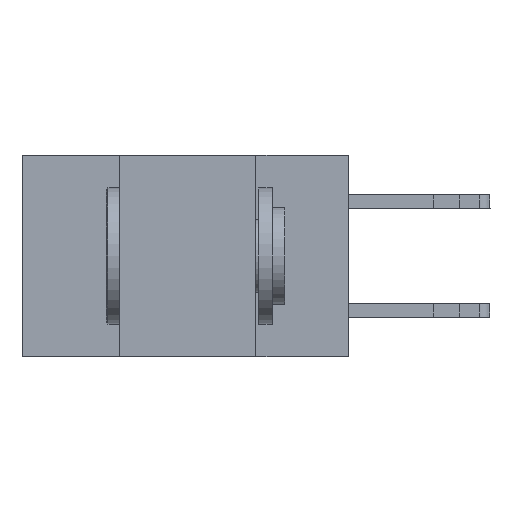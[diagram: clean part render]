
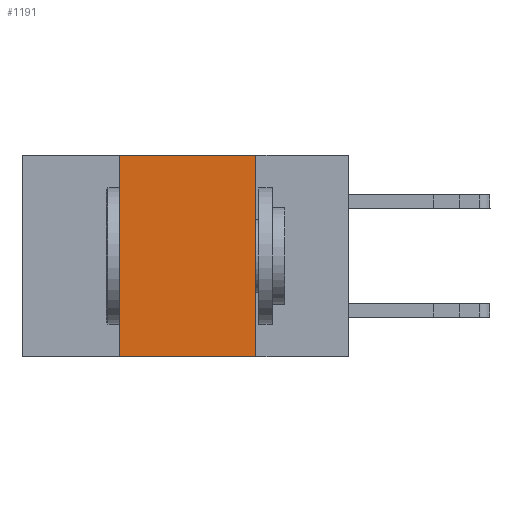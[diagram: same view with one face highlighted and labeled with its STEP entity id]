
A CAD part, left-side view. The second image highlights one B-rep face of the part: STEP entity #1191.
In plain terms, the highlighted planar face has unit normal (-1, 0, 0).
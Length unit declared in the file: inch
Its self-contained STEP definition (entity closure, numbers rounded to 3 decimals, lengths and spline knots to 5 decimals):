
#164 = ORIENTED_EDGE ( 'NONE', *, *, #8032, .T. ) ;
#178 = ORIENTED_EDGE ( 'NONE', *, *, #5772, .F. ) ;
#210 = CARTESIAN_POINT ( 'NONE',  ( 0., 0.6, 0. ) ) ;
#776 = CARTESIAN_POINT ( 'NONE',  ( 0., 0.6, 0. ) ) ;
#1191 = ADVANCED_FACE ( 'NONE', ( #9233 ), #8051, .F. ) ;
#1255 = VECTOR ( 'NONE', #7173, 39.37008 ) ;
#1764 = LINE ( 'NONE', #10640, #3026 ) ;
#2002 = VECTOR ( 'NONE', #3952, 39.37008 ) ;
#2213 = DIRECTION ( 'NONE',  ( 0., 0., -1. ) ) ;
#2550 = LINE ( 'NONE', #6993, #9428 ) ;
#2811 = CARTESIAN_POINT ( 'NONE',  ( 0., 0.17, -0.37 ) ) ;
#2927 = EDGE_LOOP ( 'NONE', ( #6967, #178, #12974, #164 ) ) ;
#3026 = VECTOR ( 'NONE', #9819, 39.37008 ) ;
#3538 = DIRECTION ( 'NONE',  ( 1., 0., 0. ) ) ;
#3952 = DIRECTION ( 'NONE',  ( 0., -1., 0. ) ) ;
#4082 = AXIS2_PLACEMENT_3D ( 'NONE', #210, #3538, #2213 ) ;
#4520 = EDGE_CURVE ( 'NONE', #13511, #6737, #2550, .T. ) ;
#5772 = EDGE_CURVE ( 'NONE', #6536, #13511, #12866, .T. ) ;
#5846 = CARTESIAN_POINT ( 'NONE',  ( 0., 0.42, 0. ) ) ;
#6536 = VERTEX_POINT ( 'NONE', #5846 ) ;
#6737 = VERTEX_POINT ( 'NONE', #2811 ) ;
#6967 = ORIENTED_EDGE ( 'NONE', *, *, #4520, .F. ) ;
#6993 = CARTESIAN_POINT ( 'NONE',  ( 0., 0.17, 0. ) ) ;
#7173 = DIRECTION ( 'NONE',  ( 0., -1., 0. ) ) ;
#8032 = EDGE_CURVE ( 'NONE', #10723, #6737, #9033, .T. ) ;
#8051 = PLANE ( 'NONE',  #4082 ) ;
#9033 = LINE ( 'NONE', #13518, #1255 ) ;
#9233 = FACE_OUTER_BOUND ( 'NONE', #2927, .T. ) ;
#9428 = VECTOR ( 'NONE', #12586, 39.37008 ) ;
#9819 = DIRECTION ( 'NONE',  ( 0., 0., 1. ) ) ;
#10640 = CARTESIAN_POINT ( 'NONE',  ( 0., 0.42, 0. ) ) ;
#10723 = VERTEX_POINT ( 'NONE', #13651 ) ;
#10919 = EDGE_CURVE ( 'NONE', #10723, #6536, #1764, .T. ) ;
#12586 = DIRECTION ( 'NONE',  ( 0., 0., -1. ) ) ;
#12866 = LINE ( 'NONE', #776, #2002 ) ;
#12974 = ORIENTED_EDGE ( 'NONE', *, *, #10919, .F. ) ;
#13511 = VERTEX_POINT ( 'NONE', #13980 ) ;
#13518 = CARTESIAN_POINT ( 'NONE',  ( 0., 0.6, -0.37 ) ) ;
#13651 = CARTESIAN_POINT ( 'NONE',  ( 0., 0.42, -0.37 ) ) ;
#13980 = CARTESIAN_POINT ( 'NONE',  ( 0., 0.17, 0. ) ) ;
